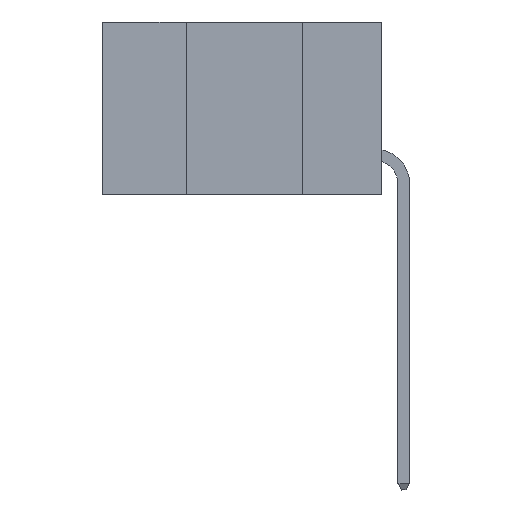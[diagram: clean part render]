
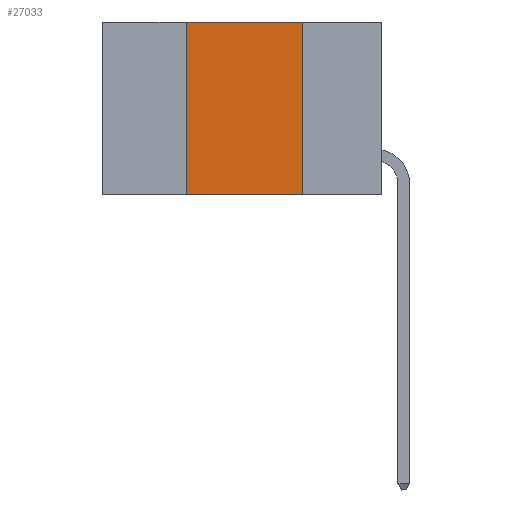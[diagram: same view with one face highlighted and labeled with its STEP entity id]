
A CAD part, left-side view. The second image highlights one B-rep face of the part: STEP entity #27033.
In plain terms, the highlighted planar face has unit normal (-1, 0, 0).
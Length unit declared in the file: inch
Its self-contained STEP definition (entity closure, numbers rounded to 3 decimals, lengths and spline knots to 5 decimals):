
#289 = VERTEX_POINT ( 'NONE', #11928 ) ;
#1583 = CARTESIAN_POINT ( 'NONE',  ( 0., 0.42, 0. ) ) ;
#1793 = CARTESIAN_POINT ( 'NONE',  ( 0., 0.6, -0.37 ) ) ;
#2978 = LINE ( 'NONE', #20622, #28963 ) ;
#3807 = ORIENTED_EDGE ( 'NONE', *, *, #31115, .F. ) ;
#3875 = VECTOR ( 'NONE', #4096, 39.37008 ) ;
#4047 = AXIS2_PLACEMENT_3D ( 'NONE', #9745, #17210, #27366 ) ;
#4096 = DIRECTION ( 'NONE',  ( 0., 0., -1. ) ) ;
#6770 = CARTESIAN_POINT ( 'NONE',  ( 0., 0.17, 0. ) ) ;
#9042 = VERTEX_POINT ( 'NONE', #1583 ) ;
#9745 = CARTESIAN_POINT ( 'NONE',  ( 0., 0.6, 0. ) ) ;
#11424 = CARTESIAN_POINT ( 'NONE',  ( 0., 0.17, 0. ) ) ;
#11928 = CARTESIAN_POINT ( 'NONE',  ( 0., 0.42, -0.37 ) ) ;
#15157 = VECTOR ( 'NONE', #30070, 39.37008 ) ;
#16508 = EDGE_CURVE ( 'NONE', #289, #19979, #16938, .T. ) ;
#16815 = VERTEX_POINT ( 'NONE', #11424 ) ;
#16938 = LINE ( 'NONE', #1793, #15157 ) ;
#17210 = DIRECTION ( 'NONE',  ( 1., 0., 0. ) ) ;
#17385 = FACE_OUTER_BOUND ( 'NONE', #30667, .T. ) ;
#19229 = PLANE ( 'NONE',  #4047 ) ;
#19979 = VERTEX_POINT ( 'NONE', #31999 ) ;
#20175 = ORIENTED_EDGE ( 'NONE', *, *, #26339, .F. ) ;
#20330 = DIRECTION ( 'NONE',  ( 0., 0., 1. ) ) ;
#20622 = CARTESIAN_POINT ( 'NONE',  ( 0., 0.6, 0. ) ) ;
#21362 = ORIENTED_EDGE ( 'NONE', *, *, #23469, .F. ) ;
#21788 = ORIENTED_EDGE ( 'NONE', *, *, #16508, .T. ) ;
#22339 = CARTESIAN_POINT ( 'NONE',  ( 0., 0.42, 0. ) ) ;
#22833 = LINE ( 'NONE', #22339, #26354 ) ;
#22951 = DIRECTION ( 'NONE',  ( 0., -1., 0. ) ) ;
#23469 = EDGE_CURVE ( 'NONE', #16815, #19979, #26887, .T. ) ;
#26339 = EDGE_CURVE ( 'NONE', #289, #9042, #22833, .T. ) ;
#26354 = VECTOR ( 'NONE', #20330, 39.37008 ) ;
#26887 = LINE ( 'NONE', #6770, #3875 ) ;
#27033 = ADVANCED_FACE ( 'NONE', ( #17385 ), #19229, .F. ) ;
#27366 = DIRECTION ( 'NONE',  ( 0., 0., -1. ) ) ;
#28963 = VECTOR ( 'NONE', #22951, 39.37008 ) ;
#30070 = DIRECTION ( 'NONE',  ( 0., -1., 0. ) ) ;
#30667 = EDGE_LOOP ( 'NONE', ( #21362, #3807, #20175, #21788 ) ) ;
#31115 = EDGE_CURVE ( 'NONE', #9042, #16815, #2978, .T. ) ;
#31999 = CARTESIAN_POINT ( 'NONE',  ( 0., 0.17, -0.37 ) ) ;
